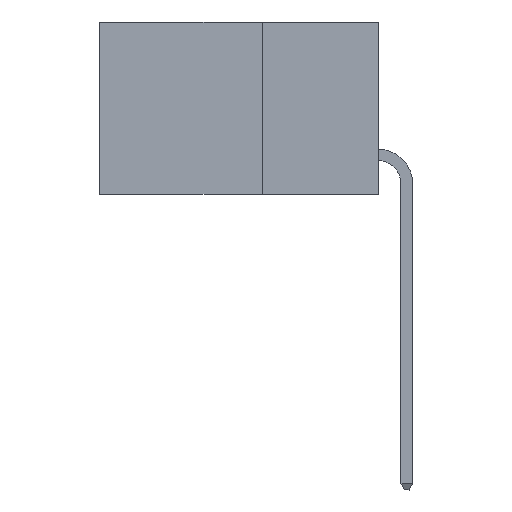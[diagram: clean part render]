
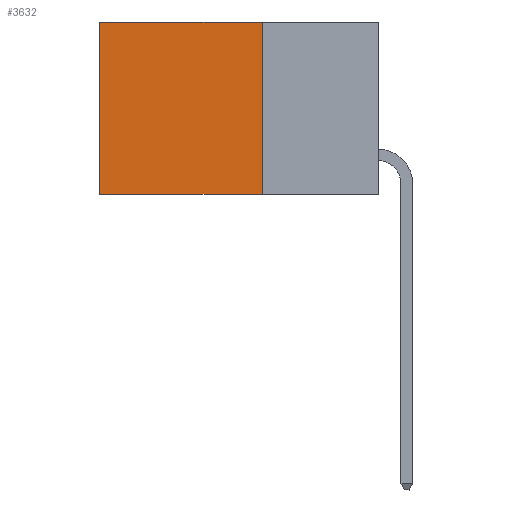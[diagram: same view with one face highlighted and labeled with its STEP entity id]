
A CAD part, left-side view. The second image highlights one B-rep face of the part: STEP entity #3632.
In plain terms, the highlighted planar face has unit normal (-1, 0, 0).
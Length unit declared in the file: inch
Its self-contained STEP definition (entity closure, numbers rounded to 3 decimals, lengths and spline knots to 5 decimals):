
#246 = DIRECTION ( 'NONE',  ( 1., 0., 0. ) ) ;
#363 = CARTESIAN_POINT ( 'NONE',  ( 0.298, 0.25, 0. ) ) ;
#1237 = LINE ( 'NONE', #10407, #14558 ) ;
#2936 = EDGE_CURVE ( 'NONE', #8886, #4602, #9134, .T. ) ;
#3066 = VERTEX_POINT ( 'NONE', #7782 ) ;
#3632 = ADVANCED_FACE ( 'NONE', ( #9671 ), #7089, .F. ) ;
#3810 = LINE ( 'NONE', #5282, #11106 ) ;
#3913 = ORIENTED_EDGE ( 'NONE', *, *, #5913, .F. ) ;
#3992 = DIRECTION ( 'NONE',  ( 0., 0., -1. ) ) ;
#4602 = VERTEX_POINT ( 'NONE', #7381 ) ;
#4931 = CARTESIAN_POINT ( 'NONE',  ( 0.298, 0.25, 0. ) ) ;
#5282 = CARTESIAN_POINT ( 'NONE',  ( 0.298, 0.6, 0. ) ) ;
#5388 = DIRECTION ( 'NONE',  ( 0., 1., 0. ) ) ;
#5564 = EDGE_CURVE ( 'NONE', #8886, #5697, #1237, .T. ) ;
#5697 = VERTEX_POINT ( 'NONE', #10770 ) ;
#5913 = EDGE_CURVE ( 'NONE', #5697, #3066, #6738, .T. ) ;
#6043 = DIRECTION ( 'NONE',  ( 0., 1., 0. ) ) ;
#6150 = EDGE_LOOP ( 'NONE', ( #9147, #3913, #13503, #14658 ) ) ;
#6738 = LINE ( 'NONE', #11046, #7285 ) ;
#7089 = PLANE ( 'NONE',  #10965 ) ;
#7285 = VECTOR ( 'NONE', #5388, 39.37008 ) ;
#7381 = CARTESIAN_POINT ( 'NONE',  ( 0.298, 0.6, 0. ) ) ;
#7782 = CARTESIAN_POINT ( 'NONE',  ( 0.298, 0.6, -0.37 ) ) ;
#7920 = VECTOR ( 'NONE', #6043, 39.37008 ) ;
#8148 = DIRECTION ( 'NONE',  ( 0., 0., -1. ) ) ;
#8303 = EDGE_CURVE ( 'NONE', #4602, #3066, #3810, .T. ) ;
#8886 = VERTEX_POINT ( 'NONE', #4931 ) ;
#9134 = LINE ( 'NONE', #9412, #7920 ) ;
#9147 = ORIENTED_EDGE ( 'NONE', *, *, #8303, .T. ) ;
#9412 = CARTESIAN_POINT ( 'NONE',  ( 0.298, 0.25, 0. ) ) ;
#9481 = DIRECTION ( 'NONE',  ( 0., 0., -1. ) ) ;
#9671 = FACE_OUTER_BOUND ( 'NONE', #6150, .T. ) ;
#10407 = CARTESIAN_POINT ( 'NONE',  ( 0.298, 0.25, 0. ) ) ;
#10770 = CARTESIAN_POINT ( 'NONE',  ( 0.298, 0.25, -0.37 ) ) ;
#10965 = AXIS2_PLACEMENT_3D ( 'NONE', #363, #246, #8148 ) ;
#11046 = CARTESIAN_POINT ( 'NONE',  ( 0.298, 0.25, -0.37 ) ) ;
#11106 = VECTOR ( 'NONE', #3992, 39.37008 ) ;
#13503 = ORIENTED_EDGE ( 'NONE', *, *, #5564, .F. ) ;
#14558 = VECTOR ( 'NONE', #9481, 39.37008 ) ;
#14658 = ORIENTED_EDGE ( 'NONE', *, *, #2936, .T. ) ;
